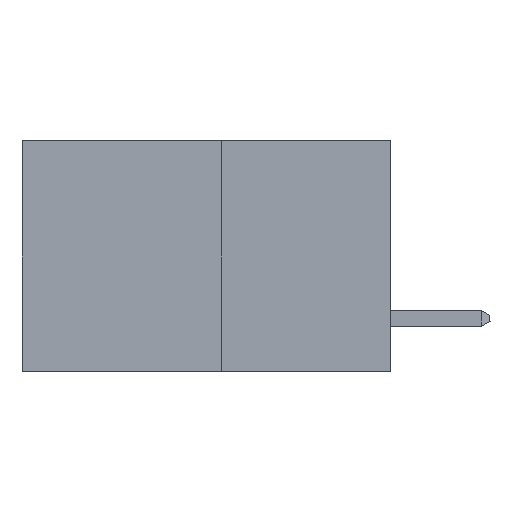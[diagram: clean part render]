
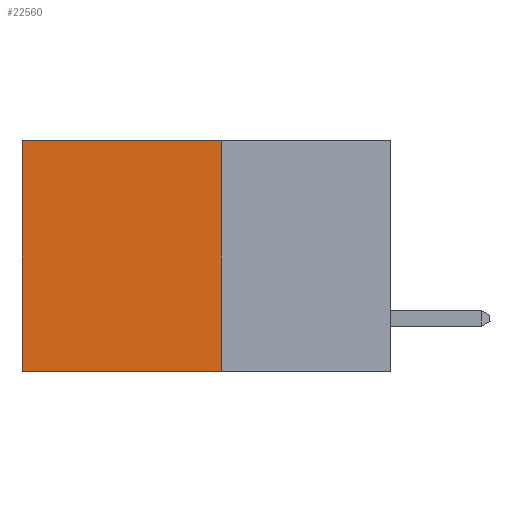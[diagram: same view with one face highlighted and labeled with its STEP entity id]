
A CAD part, left-side view. The second image highlights one B-rep face of the part: STEP entity #22560.
In plain terms, the highlighted planar face has unit normal (-1, 0, 0).
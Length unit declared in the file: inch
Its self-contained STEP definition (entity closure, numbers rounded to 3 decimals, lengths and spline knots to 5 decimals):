
#598 = FACE_OUTER_BOUND ( 'NONE', #9795, .T. ) ;
#1275 = CARTESIAN_POINT ( 'NONE',  ( 0.277, 0.59, -0.37 ) ) ;
#2957 = DIRECTION ( 'NONE',  ( 0., 0., -1. ) ) ;
#3643 = CARTESIAN_POINT ( 'NONE',  ( 0.277, 0.27, -0.37 ) ) ;
#5807 = DIRECTION ( 'NONE',  ( 0., 1., 0. ) ) ;
#6366 = LINE ( 'NONE', #3643, #16753 ) ;
#6436 = ORIENTED_EDGE ( 'NONE', *, *, #12274, .F. ) ;
#6834 = LINE ( 'NONE', #1275, #8160 ) ;
#8160 = VECTOR ( 'NONE', #19950, 39.37008 ) ;
#8659 = DIRECTION ( 'NONE',  ( 0., 0., -1. ) ) ;
#9795 = EDGE_LOOP ( 'NONE', ( #13436, #12718, #6436, #20865 ) ) ;
#10150 = LINE ( 'NONE', #23946, #15032 ) ;
#10867 = CARTESIAN_POINT ( 'NONE',  ( 0.277, 0.59, -0.37 ) ) ;
#11921 = VERTEX_POINT ( 'NONE', #16812 ) ;
#12274 = EDGE_CURVE ( 'NONE', #11921, #14542, #6366, .T. ) ;
#12718 = ORIENTED_EDGE ( 'NONE', *, *, #15398, .F. ) ;
#12725 = VECTOR ( 'NONE', #5807, 39.37008 ) ;
#12735 = CARTESIAN_POINT ( 'NONE',  ( 0.277, 0.27, -0.37 ) ) ;
#13436 = ORIENTED_EDGE ( 'NONE', *, *, #23353, .T. ) ;
#13943 = DIRECTION ( 'NONE',  ( 0., 1., 0. ) ) ;
#14542 = VERTEX_POINT ( 'NONE', #18994 ) ;
#15032 = VECTOR ( 'NONE', #13943, 39.37008 ) ;
#15398 = EDGE_CURVE ( 'NONE', #14542, #23740, #10150, .T. ) ;
#16161 = EDGE_CURVE ( 'NONE', #11921, #19457, #23438, .T. ) ;
#16753 = VECTOR ( 'NONE', #2957, 39.37008 ) ;
#16812 = CARTESIAN_POINT ( 'NONE',  ( 0.277, 0.27, 0. ) ) ;
#18936 = PLANE ( 'NONE',  #25925 ) ;
#18994 = CARTESIAN_POINT ( 'NONE',  ( 0.277, 0.27, -0.37 ) ) ;
#19457 = VERTEX_POINT ( 'NONE', #24655 ) ;
#19950 = DIRECTION ( 'NONE',  ( 0., 0., -1. ) ) ;
#20865 = ORIENTED_EDGE ( 'NONE', *, *, #16161, .T. ) ;
#20908 = DIRECTION ( 'NONE',  ( 1., 0., 0. ) ) ;
#22560 = ADVANCED_FACE ( 'NONE', ( #598 ), #18936, .F. ) ;
#23353 = EDGE_CURVE ( 'NONE', #19457, #23740, #6834, .T. ) ;
#23438 = LINE ( 'NONE', #26070, #12725 ) ;
#23740 = VERTEX_POINT ( 'NONE', #10867 ) ;
#23946 = CARTESIAN_POINT ( 'NONE',  ( 0.277, 0.27, -0.37 ) ) ;
#24655 = CARTESIAN_POINT ( 'NONE',  ( 0.277, 0.59, 0. ) ) ;
#25925 = AXIS2_PLACEMENT_3D ( 'NONE', #12735, #20908, #8659 ) ;
#26070 = CARTESIAN_POINT ( 'NONE',  ( 0.277, 0.27, 0. ) ) ;
